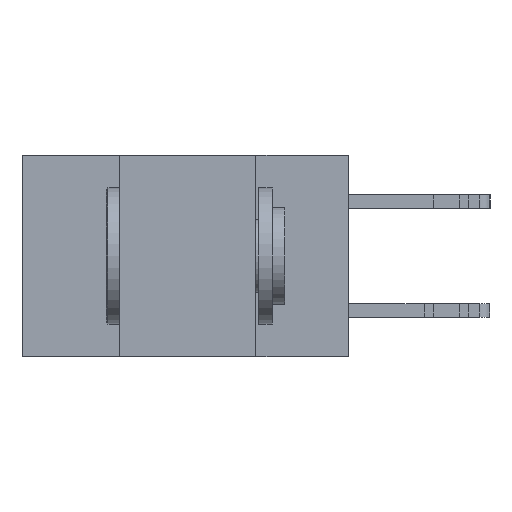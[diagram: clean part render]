
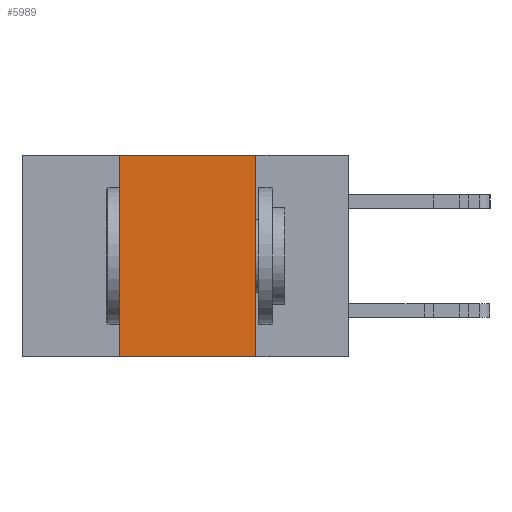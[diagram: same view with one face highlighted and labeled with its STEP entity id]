
A CAD part, left-side view. The second image highlights one B-rep face of the part: STEP entity #5989.
In plain terms, the highlighted planar face has unit normal (-1, 0, 0).
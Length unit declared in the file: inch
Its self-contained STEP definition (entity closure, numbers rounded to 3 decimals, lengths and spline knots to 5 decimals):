
#719 = VECTOR ( 'NONE', #24455, 39.37008 ) ;
#3188 = CARTESIAN_POINT ( 'NONE',  ( 0., 0.6, -0.37 ) ) ;
#4621 = EDGE_CURVE ( 'NONE', #10858, #23388, #12002, .T. ) ;
#5347 = CARTESIAN_POINT ( 'NONE',  ( 0., 0.42, -0.37 ) ) ;
#5431 = LINE ( 'NONE', #3188, #12412 ) ;
#5989 = ADVANCED_FACE ( 'NONE', ( #26064 ), #6817, .F. ) ;
#5998 = DIRECTION ( 'NONE',  ( 0., -1., 0. ) ) ;
#6817 = PLANE ( 'NONE',  #21279 ) ;
#6873 = ORIENTED_EDGE ( 'NONE', *, *, #17762, .F. ) ;
#7912 = EDGE_CURVE ( 'NONE', #24498, #10858, #21023, .T. ) ;
#8236 = CARTESIAN_POINT ( 'NONE',  ( 0., 0.17, 0. ) ) ;
#8772 = CARTESIAN_POINT ( 'NONE',  ( 0., 0.6, 0. ) ) ;
#9045 = DIRECTION ( 'NONE',  ( 1., 0., 0. ) ) ;
#9356 = EDGE_CURVE ( 'NONE', #11523, #23388, #5431, .T. ) ;
#9899 = CARTESIAN_POINT ( 'NONE',  ( 0., 0.17, -0.37 ) ) ;
#10329 = CARTESIAN_POINT ( 'NONE',  ( 0., 0.6, 0. ) ) ;
#10797 = EDGE_LOOP ( 'NONE', ( #20272, #24235, #6873, #14376 ) ) ;
#10858 = VERTEX_POINT ( 'NONE', #8236 ) ;
#10875 = DIRECTION ( 'NONE',  ( 0., 0., -1. ) ) ;
#11060 = CARTESIAN_POINT ( 'NONE',  ( 0., 0.42, 0. ) ) ;
#11183 = CARTESIAN_POINT ( 'NONE',  ( 0., 0.17, -0.37 ) ) ;
#11523 = VERTEX_POINT ( 'NONE', #22086 ) ;
#12002 = LINE ( 'NONE', #9899, #21689 ) ;
#12412 = VECTOR ( 'NONE', #20749, 39.37008 ) ;
#14160 = VECTOR ( 'NONE', #5998, 39.37008 ) ;
#14376 = ORIENTED_EDGE ( 'NONE', *, *, #9356, .T. ) ;
#17762 = EDGE_CURVE ( 'NONE', #11523, #24498, #24604, .T. ) ;
#20272 = ORIENTED_EDGE ( 'NONE', *, *, #4621, .F. ) ;
#20749 = DIRECTION ( 'NONE',  ( 0., -1., 0. ) ) ;
#21023 = LINE ( 'NONE', #10329, #14160 ) ;
#21279 = AXIS2_PLACEMENT_3D ( 'NONE', #8772, #9045, #10875 ) ;
#21689 = VECTOR ( 'NONE', #23244, 39.37008 ) ;
#22086 = CARTESIAN_POINT ( 'NONE',  ( 0., 0.42, -0.37 ) ) ;
#23244 = DIRECTION ( 'NONE',  ( 0., 0., -1. ) ) ;
#23388 = VERTEX_POINT ( 'NONE', #11183 ) ;
#24235 = ORIENTED_EDGE ( 'NONE', *, *, #7912, .F. ) ;
#24455 = DIRECTION ( 'NONE',  ( 0., 0., 1. ) ) ;
#24498 = VERTEX_POINT ( 'NONE', #11060 ) ;
#24604 = LINE ( 'NONE', #5347, #719 ) ;
#26064 = FACE_OUTER_BOUND ( 'NONE', #10797, .T. ) ;
